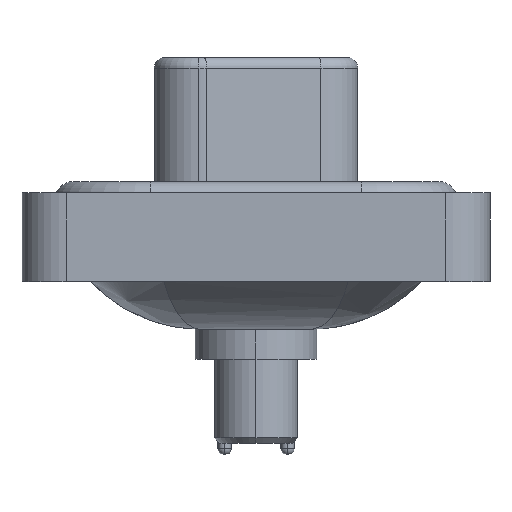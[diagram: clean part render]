
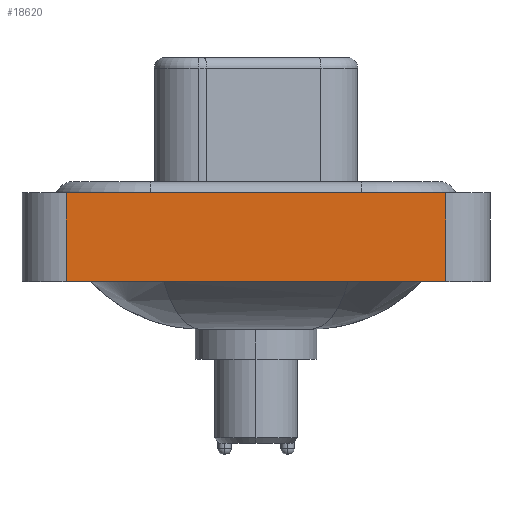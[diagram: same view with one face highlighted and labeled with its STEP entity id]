
A CAD part, left-side view. The second image highlights one B-rep face of the part: STEP entity #18620.
In plain terms, the highlighted planar face has unit normal (-1, 0, 0).
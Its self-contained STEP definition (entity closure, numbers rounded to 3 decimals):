
#82 = CARTESIAN_POINT ( 'NONE',  ( -7.3, -8.55, 0.4 ) ) ;
#1647 = DIRECTION ( 'NONE',  ( -1., 0., 0. ) ) ;
#1753 = DIRECTION ( 'NONE',  ( 0., 0., 1. ) ) ;
#2522 = CARTESIAN_POINT ( 'NONE',  ( -7.3, -8.55, -3.6 ) ) ;
#3650 = ORIENTED_EDGE ( 'NONE', *, *, #14866, .F. ) ;
#5914 = VERTEX_POINT ( 'NONE', #2522 ) ;
#6101 = DIRECTION ( 'NONE',  ( 0., -1., 0. ) ) ;
#7114 = DIRECTION ( 'NONE',  ( 0., 0., 1. ) ) ;
#7298 = LINE ( 'NONE', #13302, #16414 ) ;
#7784 = CARTESIAN_POINT ( 'NONE',  ( -7.3, -8.55, -3.6 ) ) ;
#8020 = ORIENTED_EDGE ( 'NONE', *, *, #10635, .T. ) ;
#8859 = EDGE_LOOP ( 'NONE', ( #12617, #14554, #3650, #8020 ) ) ;
#10123 = DIRECTION ( 'NONE',  ( 0., -1., 0. ) ) ;
#10635 = EDGE_CURVE ( 'NONE', #19455, #5914, #14041, .T. ) ;
#10958 = CARTESIAN_POINT ( 'NONE',  ( -7.3, 8.55, 0.4 ) ) ;
#12031 = DIRECTION ( 'NONE',  ( 0., 0., 1. ) ) ;
#12109 = FACE_OUTER_BOUND ( 'NONE', #8859, .T. ) ;
#12393 = VECTOR ( 'NONE', #10123, 1000. ) ;
#12569 = CARTESIAN_POINT ( 'NONE',  ( -7.3, -8.55, -3.6 ) ) ;
#12617 = ORIENTED_EDGE ( 'NONE', *, *, #13079, .T. ) ;
#13065 = VECTOR ( 'NONE', #7114, 1000. ) ;
#13079 = EDGE_CURVE ( 'NONE', #5914, #17685, #19044, .T. ) ;
#13302 = CARTESIAN_POINT ( 'NONE',  ( -7.3, 8.55, -3.6 ) ) ;
#13341 = EDGE_CURVE ( 'NONE', #16318, #17685, #13588, .T. ) ;
#13527 = CARTESIAN_POINT ( 'NONE',  ( -7.3, -8.55, 0.4 ) ) ;
#13588 = LINE ( 'NONE', #82, #13919 ) ;
#13919 = VECTOR ( 'NONE', #6101, 1000. ) ;
#14041 = LINE ( 'NONE', #12569, #12393 ) ;
#14554 = ORIENTED_EDGE ( 'NONE', *, *, #13341, .F. ) ;
#14707 = CARTESIAN_POINT ( 'NONE',  ( -7.3, 8.55, -3.6 ) ) ;
#14866 = EDGE_CURVE ( 'NONE', #19455, #16318, #7298, .T. ) ;
#15246 = PLANE ( 'NONE',  #15610 ) ;
#15610 = AXIS2_PLACEMENT_3D ( 'NONE', #7784, #1647, #1753 ) ;
#15981 = CARTESIAN_POINT ( 'NONE',  ( -7.3, -8.55, -3.6 ) ) ;
#16318 = VERTEX_POINT ( 'NONE', #10958 ) ;
#16414 = VECTOR ( 'NONE', #12031, 1000. ) ;
#17685 = VERTEX_POINT ( 'NONE', #13527 ) ;
#18620 = ADVANCED_FACE ( 'NONE', ( #12109 ), #15246, .T. ) ;
#19044 = LINE ( 'NONE', #15981, #13065 ) ;
#19455 = VERTEX_POINT ( 'NONE', #14707 ) ;
